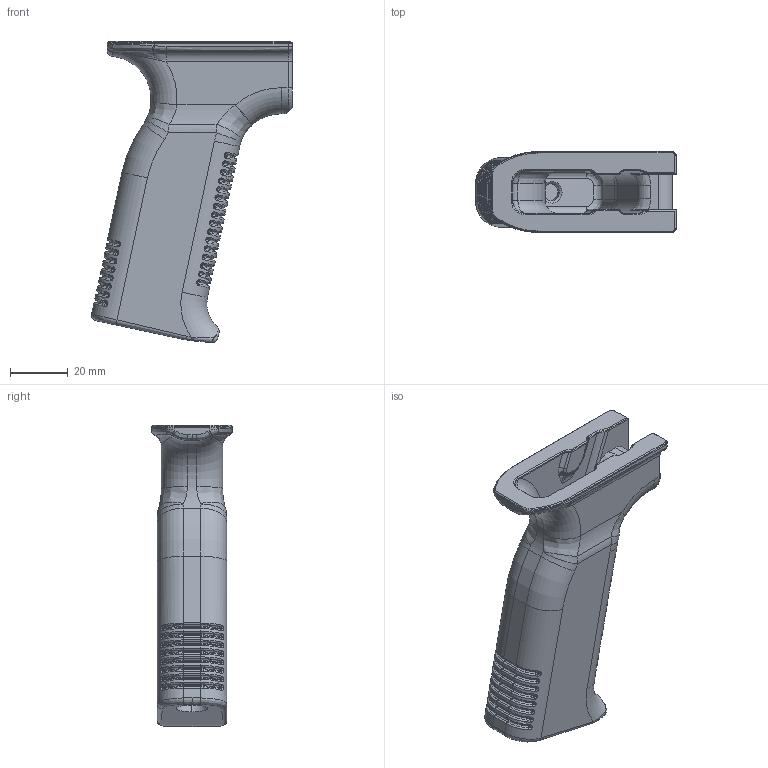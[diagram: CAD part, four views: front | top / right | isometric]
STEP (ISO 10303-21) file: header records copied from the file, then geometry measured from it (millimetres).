
FILE_DESCRIPTION(/* description */ (''),/* implementation_level */ '2;1');
FILE_NAME(/* name */ 'SureHold.step',/* time_stamp */ '2021-09-20T01:22:04-04:00',/* author */ (''),/* organization */ (''),/* preprocessor_version */ 'ST-DEVELOPER v18.1',/* originating_system */ 'Autodesk Translation Framework v10.10.0.1391',/* authorisation */ '');
FILE_SCHEMA (('AUTOMOTIVE_DESIGN { 1 0 10303 214 3 1 1 }'));
Products named in the file (1): SureHold
Bounding box: 69.45 x 28 x 104.08 mm (x, y, z)
Volume: 51243.5 mm3; surface area: 24014.5 mm2
Topology: 1 solids, 1 shells, 1278 faces, 3034 edges, 1708 vertices
Faces by surface type: bspline 468, cylinder 393, plane 198, torus 112, sphere 96, cone 11
Full cylindrical faces by diameter (mm): 14.521 x1, 16.771 x1
Entity records: 47985 total; most frequent: CARTESIAN_POINT 20842, ORIENTED_EDGE 5952, DIRECTION 5278, EDGE_CURVE 2976, AXIS2_PLACEMENT_3D 2199, VERTEX_POINT 1708, CIRCLE 1348, EDGE_LOOP 1288
